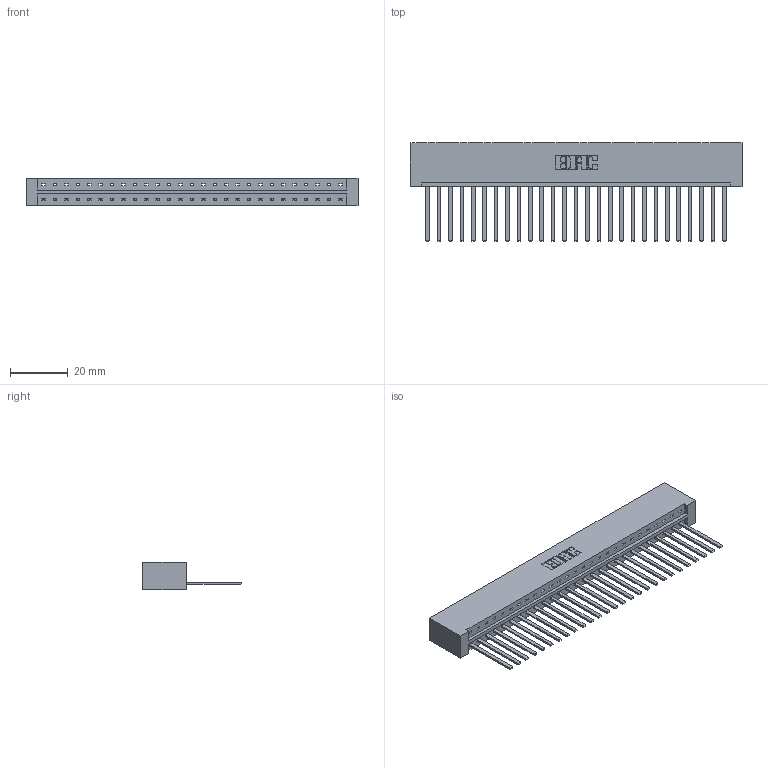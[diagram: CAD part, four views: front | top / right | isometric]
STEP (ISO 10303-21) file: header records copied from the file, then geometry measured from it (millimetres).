
FILE_DESCRIPTION (( 'STEP AP203' ), '1' );
FILE_NAME ('833-027-544-101.STEP', '2020-06-02T07:00:06', ( '' ), ( '' ), 'SwSTEP 2.0', 'SolidWorks 2020', '' );
FILE_SCHEMA (( 'CONFIG_CONTROL_DESIGN' ));
Length unit declared in the file: inch
Products named in the file (3): 833-027-544-101; 833 Part_Lugless; 345-292-001_345-293-144
Assembly tree (28 placements, depth 2):
  833-027-544-101
    833 Part_Lugless
    345-292-001_345-293-144  x27
Bounding box: 115.24 x 34.3 x 9.4 mm (x, y, z)
Volume: 12392.8 mm3; surface area: 14283.9 mm2
Topology: 28 solids, 28 shells, 1510 faces, 4553 edges, 2998 vertices
Faces by surface type: plane 1092, cylinder 418
Entity records: 17985 total; most frequent: CARTESIAN_POINT 3111, ORIENTED_EDGE 3074, DIRECTION 2643, EDGE_CURVE 1537, LINE 1421, VECTOR 1421, VERTEX_POINT 1022, AXIS2_PLACEMENT_3D 611
